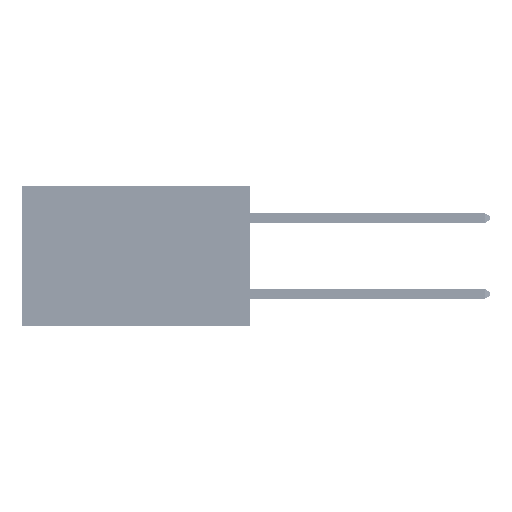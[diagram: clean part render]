
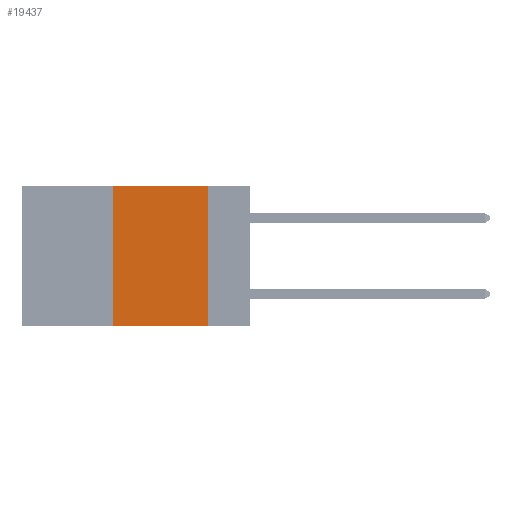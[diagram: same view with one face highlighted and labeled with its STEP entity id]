
A CAD part, left-side view. The second image highlights one B-rep face of the part: STEP entity #19437.
In plain terms, the highlighted planar face has unit normal (-1, 0, 0).
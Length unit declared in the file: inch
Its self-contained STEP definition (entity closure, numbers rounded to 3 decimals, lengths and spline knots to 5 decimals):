
#553 = EDGE_LOOP ( 'NONE', ( #43678, #15312, #43745, #5172 ) ) ;
#3125 = EDGE_CURVE ( 'NONE', #19118, #34574, #40570, .T. ) ;
#3956 = CARTESIAN_POINT ( 'NONE',  ( 0., 0.6, 0. ) ) ;
#4138 = DIRECTION ( 'NONE',  ( 0., 0., -1. ) ) ;
#4862 = CARTESIAN_POINT ( 'NONE',  ( 0., 0.36, -0.37 ) ) ;
#5043 = DIRECTION ( 'NONE',  ( 0., 0., 1. ) ) ;
#5172 = ORIENTED_EDGE ( 'NONE', *, *, #38542, .T. ) ;
#11340 = CARTESIAN_POINT ( 'NONE',  ( 0., 0.6, -0.37 ) ) ;
#13308 = CARTESIAN_POINT ( 'NONE',  ( 0., 0.36, 0. ) ) ;
#15312 = ORIENTED_EDGE ( 'NONE', *, *, #43618, .F. ) ;
#17193 = LINE ( 'NONE', #31889, #35472 ) ;
#18330 = VERTEX_POINT ( 'NONE', #13308 ) ;
#19118 = VERTEX_POINT ( 'NONE', #25229 ) ;
#19437 = ADVANCED_FACE ( 'NONE', ( #22187 ), #20087, .F. ) ;
#19824 = LINE ( 'NONE', #28764, #32398 ) ;
#20087 = PLANE ( 'NONE',  #35941 ) ;
#22187 = FACE_OUTER_BOUND ( 'NONE', #553, .T. ) ;
#25025 = CARTESIAN_POINT ( 'NONE',  ( 0., 0.11, -0.37 ) ) ;
#25229 = CARTESIAN_POINT ( 'NONE',  ( 0., 0.11, 0. ) ) ;
#28764 = CARTESIAN_POINT ( 'NONE',  ( 0., 0.36, 0. ) ) ;
#30588 = VERTEX_POINT ( 'NONE', #4862 ) ;
#31237 = DIRECTION ( 'NONE',  ( 0., -1., 0. ) ) ;
#31889 = CARTESIAN_POINT ( 'NONE',  ( 0., 0.6, 0. ) ) ;
#32398 = VECTOR ( 'NONE', #5043, 39.37008 ) ;
#34574 = VERTEX_POINT ( 'NONE', #25025 ) ;
#35472 = VECTOR ( 'NONE', #51679, 39.37008 ) ;
#35941 = AXIS2_PLACEMENT_3D ( 'NONE', #3956, #40115, #4138 ) ;
#37953 = CARTESIAN_POINT ( 'NONE',  ( 0., 0.11, 0. ) ) ;
#38542 = EDGE_CURVE ( 'NONE', #30588, #34574, #42266, .T. ) ;
#40115 = DIRECTION ( 'NONE',  ( 1., 0., 0. ) ) ;
#40570 = LINE ( 'NONE', #37953, #41836 ) ;
#41836 = VECTOR ( 'NONE', #46038, 39.37008 ) ;
#42266 = LINE ( 'NONE', #11340, #47898 ) ;
#43161 = EDGE_CURVE ( 'NONE', #30588, #18330, #19824, .T. ) ;
#43618 = EDGE_CURVE ( 'NONE', #18330, #19118, #17193, .T. ) ;
#43678 = ORIENTED_EDGE ( 'NONE', *, *, #3125, .F. ) ;
#43745 = ORIENTED_EDGE ( 'NONE', *, *, #43161, .F. ) ;
#46038 = DIRECTION ( 'NONE',  ( 0., 0., -1. ) ) ;
#47898 = VECTOR ( 'NONE', #31237, 39.37008 ) ;
#51679 = DIRECTION ( 'NONE',  ( 0., -1., 0. ) ) ;
